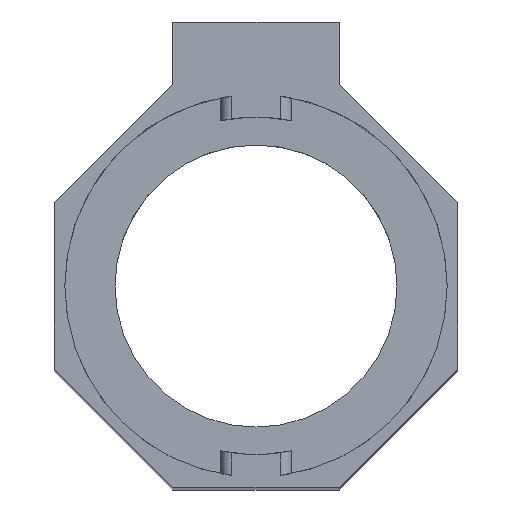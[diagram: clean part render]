
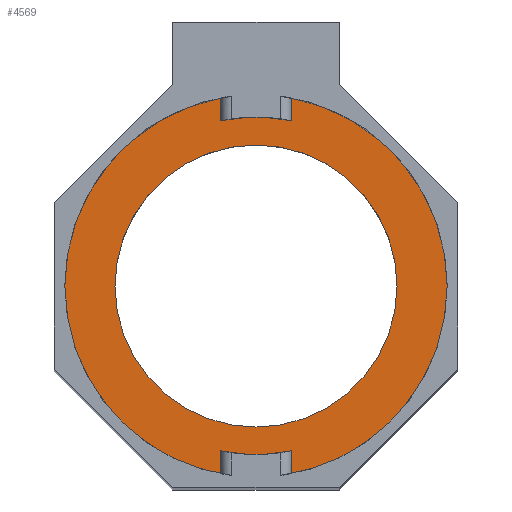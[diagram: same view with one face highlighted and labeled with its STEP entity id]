
A CAD part, top view. The second image highlights one B-rep face of the part: STEP entity #4569.
In plain terms, the highlighted planar face has unit normal (0, 0, 1).
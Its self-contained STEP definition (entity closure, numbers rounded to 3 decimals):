
#65 = VERTEX_POINT ( 'NONE', #1162 ) ;
#118 = ORIENTED_EDGE ( 'NONE', *, *, #1563, .T. ) ;
#122 = EDGE_LOOP ( 'NONE', ( #4283, #1787 ) ) ;
#283 = CIRCLE ( 'NONE', #2993, 13. ) ;
#534 = ORIENTED_EDGE ( 'NONE', *, *, #4880, .T. ) ;
#552 = EDGE_CURVE ( 'NONE', #65, #3299, #1512, .T. ) ;
#625 = AXIS2_PLACEMENT_3D ( 'NONE', #1669, #1303, #2546 ) ;
#1162 = CARTESIAN_POINT ( 'NONE',  ( -13., 0., 232.3 ) ) ;
#1192 = EDGE_LOOP ( 'NONE', ( #118, #534 ) ) ;
#1303 = DIRECTION ( 'NONE',  ( 0., 0., 1. ) ) ;
#1442 = FACE_OUTER_BOUND ( 'NONE', #1192, .T. ) ;
#1512 = CIRCLE ( 'NONE', #4223, 13. ) ;
#1563 = EDGE_CURVE ( 'NONE', #4408, #2252, #3935, .T. ) ;
#1669 = CARTESIAN_POINT ( 'NONE',  ( 0., 0., 232.3 ) ) ;
#1671 = DIRECTION ( 'NONE',  ( 0., 0., 1. ) ) ;
#1787 = ORIENTED_EDGE ( 'NONE', *, *, #2412, .F. ) ;
#1893 = CARTESIAN_POINT ( 'NONE',  ( 0., 0., 232.3 ) ) ;
#1918 = PLANE ( 'NONE',  #2790 ) ;
#2252 = VERTEX_POINT ( 'NONE', #5385 ) ;
#2412 = EDGE_CURVE ( 'NONE', #3299, #65, #283, .T. ) ;
#2546 = DIRECTION ( 'NONE',  ( 1., 0., 0. ) ) ;
#2624 = DIRECTION ( 'NONE',  ( 0., 0., 1. ) ) ;
#2710 = DIRECTION ( 'NONE',  ( 0., 0., 1. ) ) ;
#2790 = AXIS2_PLACEMENT_3D ( 'NONE', #3134, #2710, #4834 ) ;
#2931 = AXIS2_PLACEMENT_3D ( 'NONE', #1893, #3614, #4362 ) ;
#2993 = AXIS2_PLACEMENT_3D ( 'NONE', #5057, #1671, #3388 ) ;
#3134 = CARTESIAN_POINT ( 'NONE',  ( 0., 0., 232.3 ) ) ;
#3299 = VERTEX_POINT ( 'NONE', #4128 ) ;
#3388 = DIRECTION ( 'NONE',  ( 1., 0., 0. ) ) ;
#3614 = DIRECTION ( 'NONE',  ( 0., 0., 1. ) ) ;
#3695 = CIRCLE ( 'NONE', #625, 17.625 ) ;
#3865 = CARTESIAN_POINT ( 'NONE',  ( 0., 0., 232.3 ) ) ;
#3935 = CIRCLE ( 'NONE', #2931, 17.625 ) ;
#4128 = CARTESIAN_POINT ( 'NONE',  ( 13., 0., 232.3 ) ) ;
#4223 = AXIS2_PLACEMENT_3D ( 'NONE', #3865, #2624, #4769 ) ;
#4283 = ORIENTED_EDGE ( 'NONE', *, *, #552, .F. ) ;
#4362 = DIRECTION ( 'NONE',  ( 1., 0., 0. ) ) ;
#4408 = VERTEX_POINT ( 'NONE', #5516 ) ;
#4569 = ADVANCED_FACE ( 'NONE', ( #4858, #1442 ), #1918, .T. ) ;
#4769 = DIRECTION ( 'NONE',  ( 1., 0., 0. ) ) ;
#4834 = DIRECTION ( 'NONE',  ( 1., 0., 0. ) ) ;
#4858 = FACE_BOUND ( 'NONE', #122, .T. ) ;
#4880 = EDGE_CURVE ( 'NONE', #2252, #4408, #3695, .T. ) ;
#5057 = CARTESIAN_POINT ( 'NONE',  ( 0., 0., 232.3 ) ) ;
#5385 = CARTESIAN_POINT ( 'NONE',  ( -17.625, 0., 232.3 ) ) ;
#5516 = CARTESIAN_POINT ( 'NONE',  ( 17.625, 0., 232.3 ) ) ;
